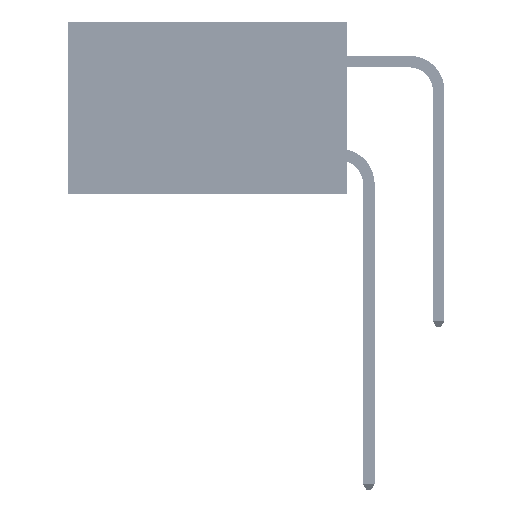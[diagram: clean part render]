
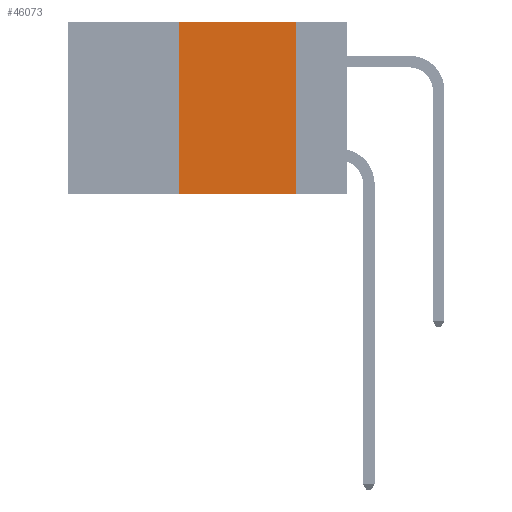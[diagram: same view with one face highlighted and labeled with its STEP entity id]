
A CAD part, left-side view. The second image highlights one B-rep face of the part: STEP entity #46073.
In plain terms, the highlighted planar face has unit normal (-1, 0, 0).
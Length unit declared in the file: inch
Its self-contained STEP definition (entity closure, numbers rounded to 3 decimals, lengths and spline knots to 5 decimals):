
#643 = EDGE_CURVE ( 'NONE', #8606, #41834, #1423, .T. ) ;
#1064 = EDGE_CURVE ( 'NONE', #31048, #25509, #3689, .T. ) ;
#1423 = LINE ( 'NONE', #7794, #30584 ) ;
#1551 = ORIENTED_EDGE ( 'NONE', *, *, #34141, .F. ) ;
#1577 = CARTESIAN_POINT ( 'NONE',  ( 0., 0.11, -0.37 ) ) ;
#3257 = LINE ( 'NONE', #38294, #12543 ) ;
#3689 = LINE ( 'NONE', #34502, #34005 ) ;
#7794 = CARTESIAN_POINT ( 'NONE',  ( 0., 0.6, -0.37 ) ) ;
#8606 = VERTEX_POINT ( 'NONE', #41181 ) ;
#9416 = DIRECTION ( 'NONE',  ( 0., 0., -1. ) ) ;
#12026 = DIRECTION ( 'NONE',  ( 0., -1., 0. ) ) ;
#12543 = VECTOR ( 'NONE', #15953, 39.37008 ) ;
#13000 = CARTESIAN_POINT ( 'NONE',  ( 0., 0.11, 0. ) ) ;
#13316 = EDGE_CURVE ( 'NONE', #25509, #41834, #30922, .T. ) ;
#13930 = ORIENTED_EDGE ( 'NONE', *, *, #643, .T. ) ;
#14855 = FACE_OUTER_BOUND ( 'NONE', #38626, .T. ) ;
#15953 = DIRECTION ( 'NONE',  ( 0., 0., 1. ) ) ;
#16067 = ORIENTED_EDGE ( 'NONE', *, *, #13316, .F. ) ;
#16622 = AXIS2_PLACEMENT_3D ( 'NONE', #29203, #44184, #36659 ) ;
#18852 = ORIENTED_EDGE ( 'NONE', *, *, #1064, .F. ) ;
#25447 = PLANE ( 'NONE',  #16622 ) ;
#25509 = VERTEX_POINT ( 'NONE', #28331 ) ;
#27109 = CARTESIAN_POINT ( 'NONE',  ( 0., 0.36, 0. ) ) ;
#27502 = DIRECTION ( 'NONE',  ( 0., -1., 0. ) ) ;
#28331 = CARTESIAN_POINT ( 'NONE',  ( 0., 0.11, 0. ) ) ;
#29203 = CARTESIAN_POINT ( 'NONE',  ( 0., 0.6, 0. ) ) ;
#30584 = VECTOR ( 'NONE', #12026, 39.37008 ) ;
#30922 = LINE ( 'NONE', #13000, #33231 ) ;
#31048 = VERTEX_POINT ( 'NONE', #27109 ) ;
#33231 = VECTOR ( 'NONE', #9416, 39.37008 ) ;
#34005 = VECTOR ( 'NONE', #27502, 39.37008 ) ;
#34141 = EDGE_CURVE ( 'NONE', #8606, #31048, #3257, .T. ) ;
#34502 = CARTESIAN_POINT ( 'NONE',  ( 0., 0.6, 0. ) ) ;
#36659 = DIRECTION ( 'NONE',  ( 0., 0., -1. ) ) ;
#38294 = CARTESIAN_POINT ( 'NONE',  ( 0., 0.36, 0. ) ) ;
#38626 = EDGE_LOOP ( 'NONE', ( #16067, #18852, #1551, #13930 ) ) ;
#41181 = CARTESIAN_POINT ( 'NONE',  ( 0., 0.36, -0.37 ) ) ;
#41834 = VERTEX_POINT ( 'NONE', #1577 ) ;
#44184 = DIRECTION ( 'NONE',  ( 1., 0., 0. ) ) ;
#46073 = ADVANCED_FACE ( 'NONE', ( #14855 ), #25447, .F. ) ;
